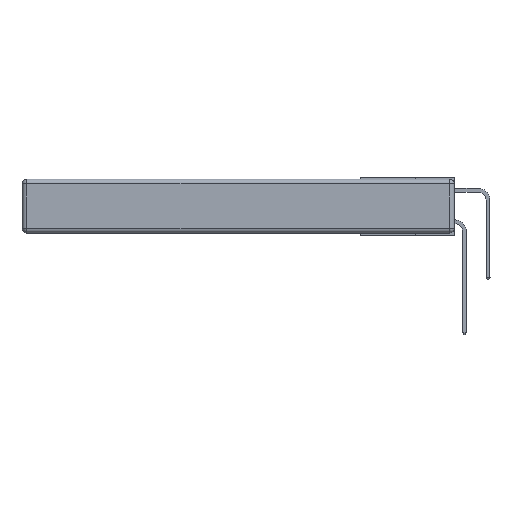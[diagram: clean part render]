
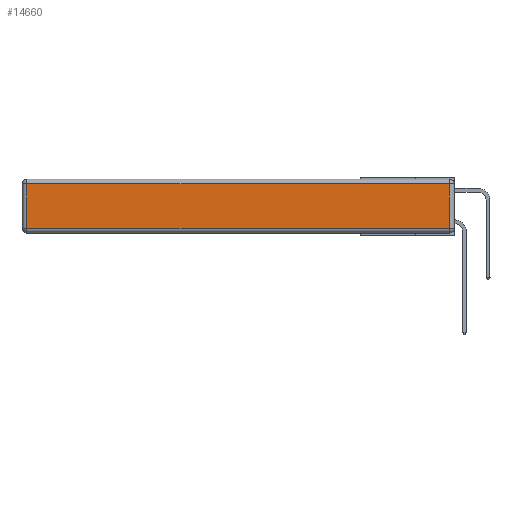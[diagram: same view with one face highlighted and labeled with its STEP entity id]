
A CAD part, left-side view. The second image highlights one B-rep face of the part: STEP entity #14660.
In plain terms, the highlighted planar face has unit normal (-1, 0, 0).
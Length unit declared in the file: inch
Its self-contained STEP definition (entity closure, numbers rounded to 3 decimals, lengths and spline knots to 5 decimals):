
#149 = EDGE_LOOP ( 'NONE', ( #4838, #13764, #5942, #764 ) ) ;
#764 = ORIENTED_EDGE ( 'NONE', *, *, #11623, .T. ) ;
#971 = DIRECTION ( 'NONE',  ( 0., 0., -1. ) ) ;
#1725 = LINE ( 'NONE', #3010, #9176 ) ;
#2137 = FACE_OUTER_BOUND ( 'NONE', #149, .T. ) ;
#3010 = CARTESIAN_POINT ( 'NONE',  ( 0., 0., -0.313 ) ) ;
#3670 = VECTOR ( 'NONE', #14039, 39.37008 ) ;
#3673 = VERTEX_POINT ( 'NONE', #11225 ) ;
#3682 = EDGE_CURVE ( 'NONE', #12975, #3673, #13541, .T. ) ;
#3841 = CARTESIAN_POINT ( 'NONE',  ( 0., 0., -0.343 ) ) ;
#3997 = VERTEX_POINT ( 'NONE', #7212 ) ;
#4582 = LINE ( 'NONE', #5836, #3670 ) ;
#4838 = ORIENTED_EDGE ( 'NONE', *, *, #9273, .T. ) ;
#5666 = CARTESIAN_POINT ( 'NONE',  ( 0., 2.72, -0.343 ) ) ;
#5836 = CARTESIAN_POINT ( 'NONE',  ( 0., 0.03, -0.343 ) ) ;
#5942 = ORIENTED_EDGE ( 'NONE', *, *, #3682, .T. ) ;
#6014 = DIRECTION ( 'NONE',  ( 0., 0., 1. ) ) ;
#6118 = PLANE ( 'NONE',  #7293 ) ;
#7212 = CARTESIAN_POINT ( 'NONE',  ( 0., 2.72, -0.313 ) ) ;
#7293 = AXIS2_PLACEMENT_3D ( 'NONE', #3841, #9568, #6014 ) ;
#7809 = CARTESIAN_POINT ( 'NONE',  ( 0., 2.75, -0.03 ) ) ;
#8032 = VECTOR ( 'NONE', #971, 39.37008 ) ;
#9176 = VECTOR ( 'NONE', #11178, 39.37008 ) ;
#9273 = EDGE_CURVE ( 'NONE', #3997, #11137, #1725, .T. ) ;
#9568 = DIRECTION ( 'NONE',  ( -1., 0., 0. ) ) ;
#10353 = CARTESIAN_POINT ( 'NONE',  ( 0., 0.03, -0.313 ) ) ;
#10384 = VECTOR ( 'NONE', #12607, 39.37008 ) ;
#10430 = CARTESIAN_POINT ( 'NONE',  ( 0., 0.03, -0.03 ) ) ;
#11137 = VERTEX_POINT ( 'NONE', #10353 ) ;
#11178 = DIRECTION ( 'NONE',  ( 0., -1., 0. ) ) ;
#11225 = CARTESIAN_POINT ( 'NONE',  ( 0., 2.72, -0.03 ) ) ;
#11623 = EDGE_CURVE ( 'NONE', #3673, #3997, #13591, .T. ) ;
#12163 = EDGE_CURVE ( 'NONE', #11137, #12975, #4582, .T. ) ;
#12607 = DIRECTION ( 'NONE',  ( 0., 1., 0. ) ) ;
#12975 = VERTEX_POINT ( 'NONE', #10430 ) ;
#13541 = LINE ( 'NONE', #7809, #10384 ) ;
#13591 = LINE ( 'NONE', #5666, #8032 ) ;
#13764 = ORIENTED_EDGE ( 'NONE', *, *, #12163, .T. ) ;
#14039 = DIRECTION ( 'NONE',  ( 0., 0., 1. ) ) ;
#14660 = ADVANCED_FACE ( 'NONE', ( #2137 ), #6118, .T. ) ;
